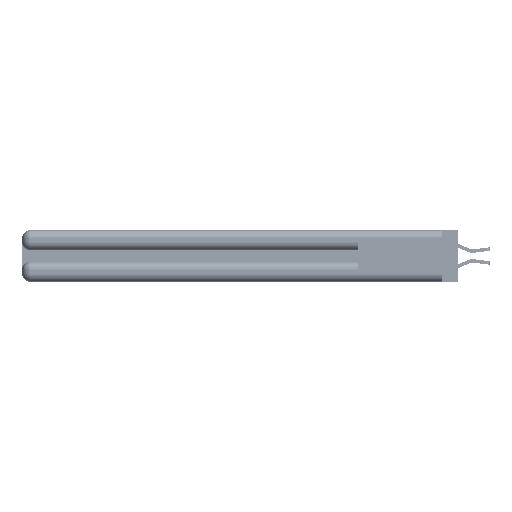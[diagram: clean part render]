
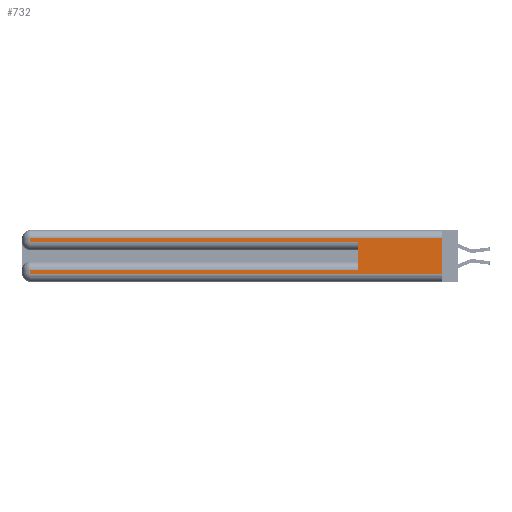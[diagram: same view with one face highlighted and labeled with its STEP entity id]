
A CAD part, left-side view. The second image highlights one B-rep face of the part: STEP entity #732.
In plain terms, the highlighted planar face has unit normal (-1, 0, 0).
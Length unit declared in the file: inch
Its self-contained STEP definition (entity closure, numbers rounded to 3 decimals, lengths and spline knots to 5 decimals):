
#732 = ADVANCED_FACE ( 'NONE', ( #41761 ), #2988, .F. ) ;
#2356 = DIRECTION ( 'NONE',  ( 0., 0., 1. ) ) ;
#2988 = PLANE ( 'NONE',  #25717 ) ;
#3264 = VERTEX_POINT ( 'NONE', #28912 ) ;
#4190 = CARTESIAN_POINT ( 'NONE',  ( 0., 0.6, 0.085 ) ) ;
#4893 = CARTESIAN_POINT ( 'NONE',  ( 0., 2.94, 0.06 ) ) ;
#5389 = VECTOR ( 'NONE', #25108, 39.37008 ) ;
#5575 = EDGE_LOOP ( 'NONE', ( #39365, #46525, #47679, #38663, #15978, #28252, #10172, #23166 ) ) ;
#6350 = VECTOR ( 'NONE', #44676, 39.37008 ) ;
#6708 = DIRECTION ( 'NONE',  ( 1., 0., 0. ) ) ;
#7506 = LINE ( 'NONE', #41002, #6350 ) ;
#9246 = LINE ( 'NONE', #11654, #37529 ) ;
#9778 = CARTESIAN_POINT ( 'NONE',  ( 0., 0.6, 0.145 ) ) ;
#10074 = EDGE_CURVE ( 'NONE', #40108, #22408, #9246, .T. ) ;
#10172 = ORIENTED_EDGE ( 'NONE', *, *, #25096, .T. ) ;
#10448 = CARTESIAN_POINT ( 'NONE',  ( 0., 0., 0.06 ) ) ;
#11654 = CARTESIAN_POINT ( 'NONE',  ( 0., 0., 0.37 ) ) ;
#12183 = DIRECTION ( 'NONE',  ( 0., -1., 0. ) ) ;
#12296 = VERTEX_POINT ( 'NONE', #18105 ) ;
#13479 = LINE ( 'NONE', #10448, #14666 ) ;
#13961 = VECTOR ( 'NONE', #20394, 39.37008 ) ;
#14295 = VERTEX_POINT ( 'NONE', #39086 ) ;
#14666 = VECTOR ( 'NONE', #36235, 39.37008 ) ;
#15067 = DIRECTION ( 'NONE',  ( 0., 1., 0. ) ) ;
#15978 = ORIENTED_EDGE ( 'NONE', *, *, #34868, .F. ) ;
#17865 = VERTEX_POINT ( 'NONE', #28954 ) ;
#18057 = EDGE_CURVE ( 'NONE', #17865, #14295, #7506, .T. ) ;
#18105 = CARTESIAN_POINT ( 'NONE',  ( 0., 0.6, 0.285 ) ) ;
#20394 = DIRECTION ( 'NONE',  ( 0., 0., -1. ) ) ;
#21423 = CARTESIAN_POINT ( 'NONE',  ( 0., 0., 0.31 ) ) ;
#22186 = VERTEX_POINT ( 'NONE', #4190 ) ;
#22408 = VERTEX_POINT ( 'NONE', #27660 ) ;
#23166 = ORIENTED_EDGE ( 'NONE', *, *, #23975, .T. ) ;
#23277 = LINE ( 'NONE', #33428, #31919 ) ;
#23975 = EDGE_CURVE ( 'NONE', #27356, #22408, #13479, .T. ) ;
#25096 = EDGE_CURVE ( 'NONE', #3264, #27356, #43350, .T. ) ;
#25108 = DIRECTION ( 'NONE',  ( 0., 1., 0. ) ) ;
#25717 = AXIS2_PLACEMENT_3D ( 'NONE', #36036, #6708, #32490 ) ;
#26756 = EDGE_CURVE ( 'NONE', #14295, #12296, #32315, .T. ) ;
#27303 = LINE ( 'NONE', #9778, #38260 ) ;
#27356 = VERTEX_POINT ( 'NONE', #4893 ) ;
#27397 = CARTESIAN_POINT ( 'NONE',  ( 0., 0., 0.31 ) ) ;
#27660 = CARTESIAN_POINT ( 'NONE',  ( 0., 0., 0.06 ) ) ;
#28252 = ORIENTED_EDGE ( 'NONE', *, *, #31796, .T. ) ;
#28912 = CARTESIAN_POINT ( 'NONE',  ( 0., 2.94, 0.085 ) ) ;
#28954 = CARTESIAN_POINT ( 'NONE',  ( 0., 2.94, 0.31 ) ) ;
#30030 = DIRECTION ( 'NONE',  ( 0., 0., -1. ) ) ;
#31155 = VECTOR ( 'NONE', #12183, 39.37008 ) ;
#31796 = EDGE_CURVE ( 'NONE', #22186, #3264, #23277, .T. ) ;
#31919 = VECTOR ( 'NONE', #15067, 39.37008 ) ;
#32315 = LINE ( 'NONE', #45184, #31155 ) ;
#32490 = DIRECTION ( 'NONE',  ( 0., 0., -1. ) ) ;
#33428 = CARTESIAN_POINT ( 'NONE',  ( 0., 0., 0.085 ) ) ;
#34787 = LINE ( 'NONE', #21423, #5389 ) ;
#34868 = EDGE_CURVE ( 'NONE', #22186, #12296, #27303, .T. ) ;
#35188 = CARTESIAN_POINT ( 'NONE',  ( 0., 2.94, 0.37 ) ) ;
#36036 = CARTESIAN_POINT ( 'NONE',  ( 0., 0., 0.37 ) ) ;
#36235 = DIRECTION ( 'NONE',  ( 0., -1., 0. ) ) ;
#37529 = VECTOR ( 'NONE', #30030, 39.37008 ) ;
#38260 = VECTOR ( 'NONE', #2356, 39.37008 ) ;
#38663 = ORIENTED_EDGE ( 'NONE', *, *, #26756, .T. ) ;
#39086 = CARTESIAN_POINT ( 'NONE',  ( 0., 2.94, 0.285 ) ) ;
#39365 = ORIENTED_EDGE ( 'NONE', *, *, #10074, .F. ) ;
#40108 = VERTEX_POINT ( 'NONE', #27397 ) ;
#41002 = CARTESIAN_POINT ( 'NONE',  ( 0., 2.94, 0.37 ) ) ;
#41761 = FACE_OUTER_BOUND ( 'NONE', #5575, .T. ) ;
#42896 = EDGE_CURVE ( 'NONE', #40108, #17865, #34787, .T. ) ;
#43350 = LINE ( 'NONE', #35188, #13961 ) ;
#44676 = DIRECTION ( 'NONE',  ( 0., 0., -1. ) ) ;
#45184 = CARTESIAN_POINT ( 'NONE',  ( 0., 0., 0.285 ) ) ;
#46525 = ORIENTED_EDGE ( 'NONE', *, *, #42896, .T. ) ;
#47679 = ORIENTED_EDGE ( 'NONE', *, *, #18057, .T. ) ;
